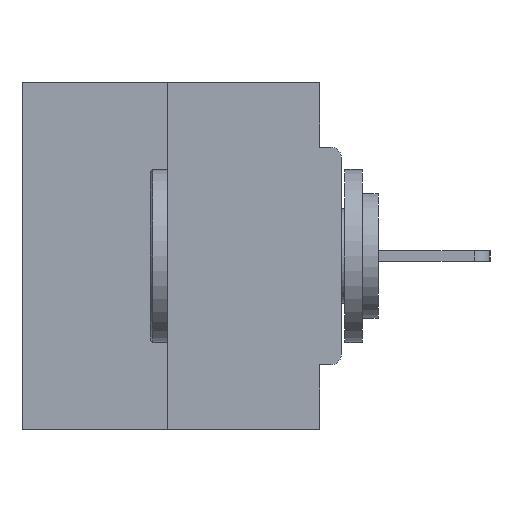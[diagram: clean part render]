
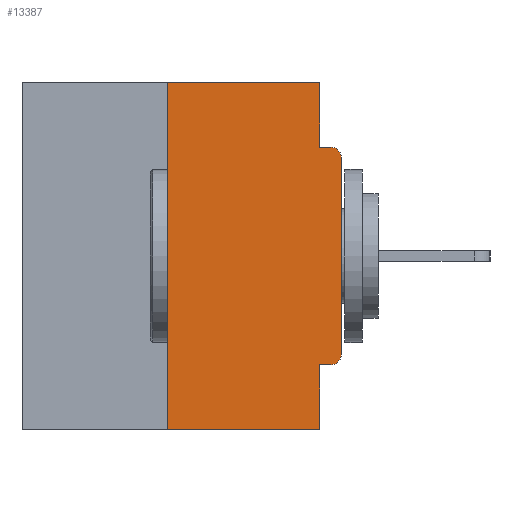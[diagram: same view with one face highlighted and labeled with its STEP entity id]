
A CAD part, left-side view. The second image highlights one B-rep face of the part: STEP entity #13387.
In plain terms, the highlighted planar face has unit normal (-1, 0, 0).
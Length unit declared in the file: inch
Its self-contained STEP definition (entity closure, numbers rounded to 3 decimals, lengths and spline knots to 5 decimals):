
#107 = VERTEX_POINT ( 'NONE', #17588 ) ;
#254 = CARTESIAN_POINT ( 'NONE',  ( 0., 0.015, -0.3915 ) ) ;
#282 = EDGE_LOOP ( 'NONE', ( #13273, #1290, #26545, #22257, #6249, #20311, #11522, #8585, #12057, #6518 ) ) ;
#715 = EDGE_CURVE ( 'NONE', #22937, #8027, #3657, .T. ) ;
#981 = VERTEX_POINT ( 'NONE', #11760 ) ;
#1064 = VERTEX_POINT ( 'NONE', #18800 ) ;
#1290 = ORIENTED_EDGE ( 'NONE', *, *, #19329, .F. ) ;
#1332 = EDGE_CURVE ( 'NONE', #107, #22937, #24674, .T. ) ;
#1644 = LINE ( 'NONE', #3754, #7559 ) ;
#2172 = VECTOR ( 'NONE', #12104, 39.37008 ) ;
#2229 = EDGE_CURVE ( 'NONE', #107, #26118, #13233, .T. ) ;
#3657 = LINE ( 'NONE', #10743, #15245 ) ;
#3754 = CARTESIAN_POINT ( 'NONE',  ( 0., 0., 0. ) ) ;
#3813 = DIRECTION ( 'NONE',  ( 0., 0., -1. ) ) ;
#3897 = EDGE_CURVE ( 'NONE', #1064, #26020, #26876, .T. ) ;
#5318 = CARTESIAN_POINT ( 'NONE',  ( 0., 0.031, 0. ) ) ;
#5375 = EDGE_CURVE ( 'NONE', #26118, #26004, #1644, .T. ) ;
#5761 = CARTESIAN_POINT ( 'NONE',  ( 0., 0., -0.3915 ) ) ;
#5960 = AXIS2_PLACEMENT_3D ( 'NONE', #11503, #16572, #14330 ) ;
#6249 = ORIENTED_EDGE ( 'NONE', *, *, #1332, .F. ) ;
#6518 = ORIENTED_EDGE ( 'NONE', *, *, #8899, .F. ) ;
#7559 = VECTOR ( 'NONE', #19833, 39.37008 ) ;
#8027 = VERTEX_POINT ( 'NONE', #16846 ) ;
#8089 = DIRECTION ( 'NONE',  ( 0., -1., 0. ) ) ;
#8585 = ORIENTED_EDGE ( 'NONE', *, *, #25945, .T. ) ;
#8899 = EDGE_CURVE ( 'NONE', #26020, #17289, #12408, .T. ) ;
#9126 = DIRECTION ( 'NONE',  ( 0., -1., 0. ) ) ;
#9132 = CARTESIAN_POINT ( 'NONE',  ( 0., 0.031, -0.4065 ) ) ;
#9448 = DIRECTION ( 'NONE',  ( 0., 0., -1. ) ) ;
#9845 = AXIS2_PLACEMENT_3D ( 'NONE', #17274, #12952, #12646 ) ;
#9981 = CARTESIAN_POINT ( 'NONE',  ( 0., 0., -0.1085 ) ) ;
#10743 = CARTESIAN_POINT ( 'NONE',  ( 0., 0.031, -0.5 ) ) ;
#10849 = DIRECTION ( 'NONE',  ( 0., 1., 0. ) ) ;
#11503 = CARTESIAN_POINT ( 'NONE',  ( 0., 0.015, -0.1085 ) ) ;
#11522 = ORIENTED_EDGE ( 'NONE', *, *, #5375, .T. ) ;
#11760 = CARTESIAN_POINT ( 'NONE',  ( 0., 0.015, -0.0935 ) ) ;
#12057 = ORIENTED_EDGE ( 'NONE', *, *, #28360, .F. ) ;
#12104 = DIRECTION ( 'NONE',  ( 0., 0., -1. ) ) ;
#12408 = LINE ( 'NONE', #5318, #2172 ) ;
#12628 = CARTESIAN_POINT ( 'NONE',  ( 0., 0., -0.0935 ) ) ;
#12646 = DIRECTION ( 'NONE',  ( 0., 0., -1. ) ) ;
#12952 = DIRECTION ( 'NONE',  ( 1., 0., 0. ) ) ;
#13233 = CIRCLE ( 'NONE', #25216, 0.015 ) ;
#13273 = ORIENTED_EDGE ( 'NONE', *, *, #3897, .F. ) ;
#13387 = ADVANCED_FACE ( 'NONE', ( #17576 ), #15490, .F. ) ;
#14330 = DIRECTION ( 'NONE',  ( 0., 0., -1. ) ) ;
#14655 = CARTESIAN_POINT ( 'NONE',  ( 0., 0.031, -0.0935 ) ) ;
#15245 = VECTOR ( 'NONE', #3813, 39.37008 ) ;
#15447 = CARTESIAN_POINT ( 'NONE',  ( 0., 0.46, 0. ) ) ;
#15490 = PLANE ( 'NONE',  #9845 ) ;
#16133 = VECTOR ( 'NONE', #9126, 39.37008 ) ;
#16572 = DIRECTION ( 'NONE',  ( -1., 0., 0. ) ) ;
#16846 = CARTESIAN_POINT ( 'NONE',  ( 0., 0.031, -0.5 ) ) ;
#17274 = CARTESIAN_POINT ( 'NONE',  ( 0., 0.46, 0. ) ) ;
#17289 = VERTEX_POINT ( 'NONE', #14655 ) ;
#17299 = CARTESIAN_POINT ( 'NONE',  ( 0., 0.25, 0. ) ) ;
#17576 = FACE_OUTER_BOUND ( 'NONE', #282, .T. ) ;
#17588 = CARTESIAN_POINT ( 'NONE',  ( 0., 0.015, -0.4065 ) ) ;
#18154 = LINE ( 'NONE', #29616, #22469 ) ;
#18800 = CARTESIAN_POINT ( 'NONE',  ( 0., 0.25, 0. ) ) ;
#18882 = CIRCLE ( 'NONE', #5960, 0.015 ) ;
#18952 = DIRECTION ( 'NONE',  ( 0., 0., 1. ) ) ;
#19219 = EDGE_CURVE ( 'NONE', #21125, #8027, #18154, .T. ) ;
#19329 = EDGE_CURVE ( 'NONE', #21125, #1064, #19563, .T. ) ;
#19563 = LINE ( 'NONE', #17299, #20054 ) ;
#19833 = DIRECTION ( 'NONE',  ( 0., 0., 1. ) ) ;
#20054 = VECTOR ( 'NONE', #18952, 39.37008 ) ;
#20311 = ORIENTED_EDGE ( 'NONE', *, *, #2229, .T. ) ;
#21125 = VERTEX_POINT ( 'NONE', #24405 ) ;
#22257 = ORIENTED_EDGE ( 'NONE', *, *, #715, .F. ) ;
#22380 = VECTOR ( 'NONE', #10849, 39.37008 ) ;
#22412 = CARTESIAN_POINT ( 'NONE',  ( 0., 0., -0.4065 ) ) ;
#22469 = VECTOR ( 'NONE', #22825, 39.37008 ) ;
#22825 = DIRECTION ( 'NONE',  ( 0., -1., 0. ) ) ;
#22831 = DIRECTION ( 'NONE',  ( -1., 0., 0. ) ) ;
#22937 = VERTEX_POINT ( 'NONE', #9132 ) ;
#24184 = LINE ( 'NONE', #12628, #28390 ) ;
#24405 = CARTESIAN_POINT ( 'NONE',  ( 0., 0.25, -0.5 ) ) ;
#24674 = LINE ( 'NONE', #22412, #22380 ) ;
#25216 = AXIS2_PLACEMENT_3D ( 'NONE', #254, #22831, #9448 ) ;
#25945 = EDGE_CURVE ( 'NONE', #26004, #981, #18882, .T. ) ;
#26004 = VERTEX_POINT ( 'NONE', #9981 ) ;
#26020 = VERTEX_POINT ( 'NONE', #28770 ) ;
#26118 = VERTEX_POINT ( 'NONE', #5761 ) ;
#26545 = ORIENTED_EDGE ( 'NONE', *, *, #19219, .T. ) ;
#26876 = LINE ( 'NONE', #15447, #16133 ) ;
#28360 = EDGE_CURVE ( 'NONE', #17289, #981, #24184, .T. ) ;
#28390 = VECTOR ( 'NONE', #8089, 39.37008 ) ;
#28770 = CARTESIAN_POINT ( 'NONE',  ( 0., 0.031, 0. ) ) ;
#29616 = CARTESIAN_POINT ( 'NONE',  ( 0., 0.46, -0.5 ) ) ;
